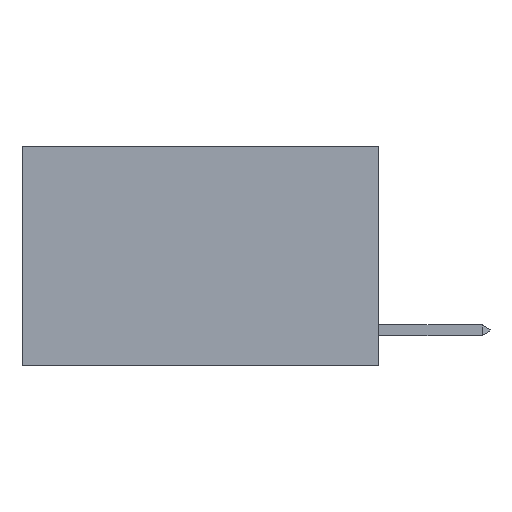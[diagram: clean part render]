
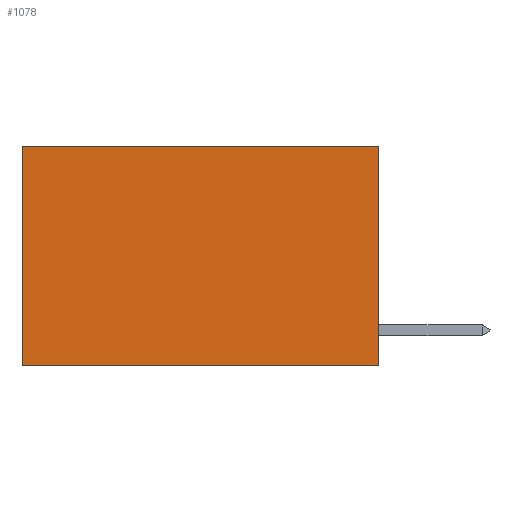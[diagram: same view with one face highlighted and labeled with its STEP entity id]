
A CAD part, left-side view. The second image highlights one B-rep face of the part: STEP entity #1078.
In plain terms, the highlighted planar face has unit normal (-1, 0, 0).
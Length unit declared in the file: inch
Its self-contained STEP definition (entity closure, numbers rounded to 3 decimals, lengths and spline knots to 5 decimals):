
#147 = EDGE_CURVE ( 'NONE', #3629, #366, #2297, .T. ) ;
#162 = CARTESIAN_POINT ( 'NONE',  ( 0.2625, 0., -0.37 ) ) ;
#366 = VERTEX_POINT ( 'NONE', #9028 ) ;
#734 = LINE ( 'NONE', #2831, #9623 ) ;
#1078 = ADVANCED_FACE ( 'NONE', ( #9633 ), #8101, .F. ) ;
#1130 = DIRECTION ( 'NONE',  ( 0., 0., -1. ) ) ;
#1231 = DIRECTION ( 'NONE',  ( 0., 0., -1. ) ) ;
#1341 = EDGE_CURVE ( 'NONE', #4781, #4313, #734, .T. ) ;
#2085 = CARTESIAN_POINT ( 'NONE',  ( 0.2625, 0., 0. ) ) ;
#2297 = LINE ( 'NONE', #8092, #4014 ) ;
#2826 = LINE ( 'NONE', #162, #7508 ) ;
#2831 = CARTESIAN_POINT ( 'NONE',  ( 0.2625, 0.6, 0. ) ) ;
#3629 = VERTEX_POINT ( 'NONE', #2085 ) ;
#3793 = ORIENTED_EDGE ( 'NONE', *, *, #1341, .T. ) ;
#3904 = ORIENTED_EDGE ( 'NONE', *, *, #4919, .F. ) ;
#4014 = VECTOR ( 'NONE', #1130, 39.37008 ) ;
#4026 = LINE ( 'NONE', #9421, #10227 ) ;
#4067 = ORIENTED_EDGE ( 'NONE', *, *, #147, .F. ) ;
#4111 = ORIENTED_EDGE ( 'NONE', *, *, #8542, .T. ) ;
#4313 = VERTEX_POINT ( 'NONE', #7684 ) ;
#4781 = VERTEX_POINT ( 'NONE', #7586 ) ;
#4919 = EDGE_CURVE ( 'NONE', #366, #4313, #2826, .T. ) ;
#5946 = DIRECTION ( 'NONE',  ( 0., 0., -1. ) ) ;
#5993 = DIRECTION ( 'NONE',  ( 1., 0., 0. ) ) ;
#7508 = VECTOR ( 'NONE', #8312, 39.37008 ) ;
#7586 = CARTESIAN_POINT ( 'NONE',  ( 0.2625, 0.6, 0. ) ) ;
#7684 = CARTESIAN_POINT ( 'NONE',  ( 0.2625, 0.6, -0.37 ) ) ;
#7767 = DIRECTION ( 'NONE',  ( 0., 1., 0. ) ) ;
#8092 = CARTESIAN_POINT ( 'NONE',  ( 0.2625, 0., 0. ) ) ;
#8096 = EDGE_LOOP ( 'NONE', ( #3793, #3904, #4067, #4111 ) ) ;
#8101 = PLANE ( 'NONE',  #10674 ) ;
#8312 = DIRECTION ( 'NONE',  ( 0., 1., 0. ) ) ;
#8542 = EDGE_CURVE ( 'NONE', #3629, #4781, #4026, .T. ) ;
#8929 = CARTESIAN_POINT ( 'NONE',  ( 0.2625, 0., 0. ) ) ;
#9028 = CARTESIAN_POINT ( 'NONE',  ( 0.2625, 0., -0.37 ) ) ;
#9421 = CARTESIAN_POINT ( 'NONE',  ( 0.2625, 0., 0. ) ) ;
#9623 = VECTOR ( 'NONE', #1231, 39.37008 ) ;
#9633 = FACE_OUTER_BOUND ( 'NONE', #8096, .T. ) ;
#10227 = VECTOR ( 'NONE', #7767, 39.37008 ) ;
#10674 = AXIS2_PLACEMENT_3D ( 'NONE', #8929, #5993, #5946 ) ;
